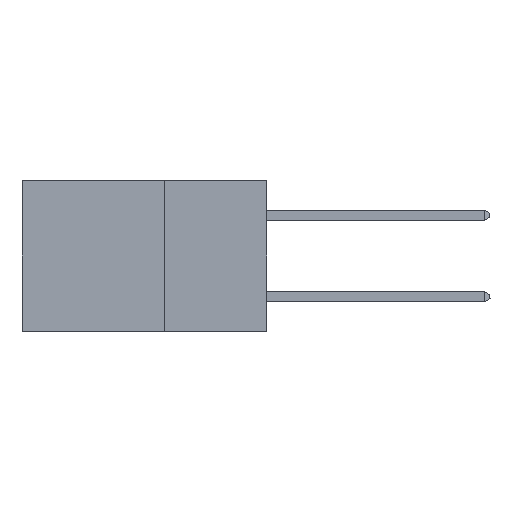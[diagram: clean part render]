
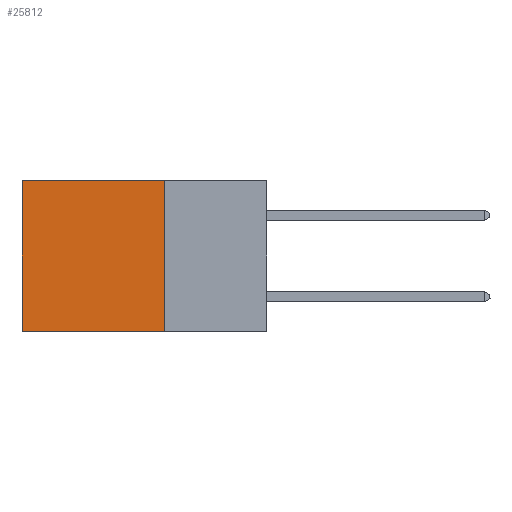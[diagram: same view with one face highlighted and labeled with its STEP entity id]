
A CAD part, left-side view. The second image highlights one B-rep face of the part: STEP entity #25812.
In plain terms, the highlighted planar face has unit normal (-1, 0, 0).
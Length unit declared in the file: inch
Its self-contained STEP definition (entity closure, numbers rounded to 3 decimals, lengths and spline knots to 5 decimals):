
#706 = EDGE_CURVE ( 'NONE', #10521, #22484, #1367, .T. ) ;
#1367 = LINE ( 'NONE', #7310, #6930 ) ;
#3395 = DIRECTION ( 'NONE',  ( 0., 0., -1. ) ) ;
#5783 = CARTESIAN_POINT ( 'NONE',  ( 0.2875, 0.25, 0. ) ) ;
#6401 = DIRECTION ( 'NONE',  ( 1., 0., 0. ) ) ;
#6679 = ORIENTED_EDGE ( 'NONE', *, *, #16256, .F. ) ;
#6930 = VECTOR ( 'NONE', #3395, 39.37008 ) ;
#7310 = CARTESIAN_POINT ( 'NONE',  ( 0.2875, 0.6, 0. ) ) ;
#7658 = EDGE_CURVE ( 'NONE', #15701, #24751, #24805, .T. ) ;
#7910 = EDGE_LOOP ( 'NONE', ( #22842, #6679, #9209, #10780 ) ) ;
#8336 = DIRECTION ( 'NONE',  ( 0., 1., 0. ) ) ;
#8721 = EDGE_CURVE ( 'NONE', #15701, #10521, #11301, .T. ) ;
#9209 = ORIENTED_EDGE ( 'NONE', *, *, #7658, .F. ) ;
#9300 = CARTESIAN_POINT ( 'NONE',  ( 0.2875, 0.25, -0.37 ) ) ;
#9742 = LINE ( 'NONE', #24303, #12250 ) ;
#10074 = CARTESIAN_POINT ( 'NONE',  ( 0.2875, 0.6, -0.37 ) ) ;
#10521 = VERTEX_POINT ( 'NONE', #25321 ) ;
#10780 = ORIENTED_EDGE ( 'NONE', *, *, #8721, .T. ) ;
#11301 = LINE ( 'NONE', #5783, #13808 ) ;
#12250 = VECTOR ( 'NONE', #8336, 39.37008 ) ;
#13808 = VECTOR ( 'NONE', #21654, 39.37008 ) ;
#14301 = PLANE ( 'NONE',  #23237 ) ;
#15701 = VERTEX_POINT ( 'NONE', #18411 ) ;
#16256 = EDGE_CURVE ( 'NONE', #24751, #22484, #9742, .T. ) ;
#16357 = CARTESIAN_POINT ( 'NONE',  ( 0.2875, 0.25, 0. ) ) ;
#17694 = CARTESIAN_POINT ( 'NONE',  ( 0.2875, 0.25, 0. ) ) ;
#18250 = FACE_OUTER_BOUND ( 'NONE', #7910, .T. ) ;
#18411 = CARTESIAN_POINT ( 'NONE',  ( 0.2875, 0.25, 0. ) ) ;
#20352 = DIRECTION ( 'NONE',  ( 0., 0., -1. ) ) ;
#21613 = DIRECTION ( 'NONE',  ( 0., 0., -1. ) ) ;
#21654 = DIRECTION ( 'NONE',  ( 0., 1., 0. ) ) ;
#22484 = VERTEX_POINT ( 'NONE', #10074 ) ;
#22842 = ORIENTED_EDGE ( 'NONE', *, *, #706, .T. ) ;
#23237 = AXIS2_PLACEMENT_3D ( 'NONE', #16357, #6401, #20352 ) ;
#24303 = CARTESIAN_POINT ( 'NONE',  ( 0.2875, 0.25, -0.37 ) ) ;
#24751 = VERTEX_POINT ( 'NONE', #9300 ) ;
#24805 = LINE ( 'NONE', #17694, #25137 ) ;
#25137 = VECTOR ( 'NONE', #21613, 39.37008 ) ;
#25321 = CARTESIAN_POINT ( 'NONE',  ( 0.2875, 0.6, 0. ) ) ;
#25812 = ADVANCED_FACE ( 'NONE', ( #18250 ), #14301, .F. ) ;
